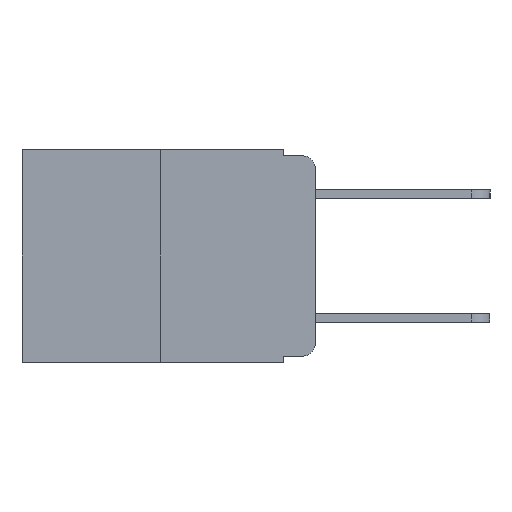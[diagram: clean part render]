
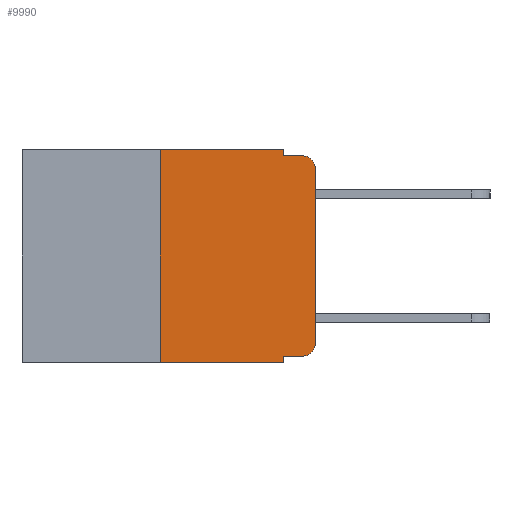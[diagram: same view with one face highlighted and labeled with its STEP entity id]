
A CAD part, left-side view. The second image highlights one B-rep face of the part: STEP entity #9990.
In plain terms, the highlighted planar face has unit normal (-1, 0, 0).
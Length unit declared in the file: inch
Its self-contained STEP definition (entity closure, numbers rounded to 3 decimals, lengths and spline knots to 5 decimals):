
#39 = VECTOR ( 'NONE', #6651, 39.37008 ) ;
#252 = EDGE_CURVE ( 'NONE', #6690, #4127, #8636, .T. ) ;
#424 = ORIENTED_EDGE ( 'NONE', *, *, #975, .F. ) ;
#566 = CARTESIAN_POINT ( 'NONE',  ( 0., 0.051, -0.333 ) ) ;
#813 = VERTEX_POINT ( 'NONE', #3341 ) ;
#815 = CARTESIAN_POINT ( 'NONE',  ( 0., 0.051, -0.343 ) ) ;
#975 = EDGE_CURVE ( 'NONE', #4862, #4857, #8998, .T. ) ;
#1001 = DIRECTION ( 'NONE',  ( 0., 0., -1. ) ) ;
#1686 = CARTESIAN_POINT ( 'NONE',  ( 0., 0.02, -0.01 ) ) ;
#1815 = EDGE_CURVE ( 'NONE', #7677, #4127, #7335, .T. ) ;
#1852 = DIRECTION ( 'NONE',  ( 0., -1., 0. ) ) ;
#1937 = CARTESIAN_POINT ( 'NONE',  ( 0., 0.051, 0. ) ) ;
#2047 = DIRECTION ( 'NONE',  ( 0., -1., 0. ) ) ;
#2063 = VECTOR ( 'NONE', #2047, 39.37008 ) ;
#2156 = CARTESIAN_POINT ( 'NONE',  ( 0., 0.051, -0.01 ) ) ;
#2443 = EDGE_CURVE ( 'NONE', #5878, #5564, #2507, .T. ) ;
#2507 = LINE ( 'NONE', #6646, #39 ) ;
#2585 = ORIENTED_EDGE ( 'NONE', *, *, #8378, .F. ) ;
#2868 = CARTESIAN_POINT ( 'NONE',  ( 0., 0., -0.03 ) ) ;
#2990 = VERTEX_POINT ( 'NONE', #2156 ) ;
#3038 = VERTEX_POINT ( 'NONE', #1686 ) ;
#3105 = AXIS2_PLACEMENT_3D ( 'NONE', #7764, #5228, #10895 ) ;
#3159 = DIRECTION ( 'NONE',  ( 0., 0., 1. ) ) ;
#3266 = CARTESIAN_POINT ( 'NONE',  ( 0., 0.25, 0. ) ) ;
#3341 = CARTESIAN_POINT ( 'NONE',  ( 0., 0.02, -0.333 ) ) ;
#3349 = VECTOR ( 'NONE', #1852, 39.37008 ) ;
#3759 = ORIENTED_EDGE ( 'NONE', *, *, #6313, .T. ) ;
#3770 = CARTESIAN_POINT ( 'NONE',  ( 0., 0.051, -0.01 ) ) ;
#3974 = CARTESIAN_POINT ( 'NONE',  ( 0., 0.051, -0.333 ) ) ;
#4127 = VERTEX_POINT ( 'NONE', #815 ) ;
#4305 = LINE ( 'NONE', #10656, #8768 ) ;
#4346 = EDGE_CURVE ( 'NONE', #6690, #813, #10275, .T. ) ;
#4380 = EDGE_LOOP ( 'NONE', ( #8405, #6462, #4447, #2585, #424, #5248, #9637, #9890, #5779, #3759 ) ) ;
#4447 = ORIENTED_EDGE ( 'NONE', *, *, #6150, .F. ) ;
#4481 = LINE ( 'NONE', #3770, #2063 ) ;
#4497 = CARTESIAN_POINT ( 'NONE',  ( 0., 0.02, -0.03 ) ) ;
#4857 = VERTEX_POINT ( 'NONE', #5536 ) ;
#4862 = VERTEX_POINT ( 'NONE', #9070 ) ;
#5085 = EDGE_CURVE ( 'NONE', #5564, #3038, #6872, .T. ) ;
#5193 = EDGE_CURVE ( 'NONE', #7677, #4862, #8290, .T. ) ;
#5228 = DIRECTION ( 'NONE',  ( 1., 0., 0. ) ) ;
#5248 = ORIENTED_EDGE ( 'NONE', *, *, #5193, .F. ) ;
#5331 = CARTESIAN_POINT ( 'NONE',  ( 0., 0.473, -0.343 ) ) ;
#5333 = VECTOR ( 'NONE', #5379, 39.37008 ) ;
#5379 = DIRECTION ( 'NONE',  ( 0., -1., 0. ) ) ;
#5536 = CARTESIAN_POINT ( 'NONE',  ( 0., 0.051, 0. ) ) ;
#5564 = VERTEX_POINT ( 'NONE', #2868 ) ;
#5629 = DIRECTION ( 'NONE',  ( -1., 0., 0. ) ) ;
#5668 = DIRECTION ( 'NONE',  ( 0., 0., -1. ) ) ;
#5779 = ORIENTED_EDGE ( 'NONE', *, *, #4346, .T. ) ;
#5878 = VERTEX_POINT ( 'NONE', #6399 ) ;
#6150 = EDGE_CURVE ( 'NONE', #2990, #3038, #4481, .T. ) ;
#6313 = EDGE_CURVE ( 'NONE', #813, #5878, #10624, .T. ) ;
#6352 = DIRECTION ( 'NONE',  ( 0., 0., -1. ) ) ;
#6399 = CARTESIAN_POINT ( 'NONE',  ( 0., 0., -0.313 ) ) ;
#6462 = ORIENTED_EDGE ( 'NONE', *, *, #5085, .T. ) ;
#6646 = CARTESIAN_POINT ( 'NONE',  ( 0., 0., 0. ) ) ;
#6651 = DIRECTION ( 'NONE',  ( 0., 0., 1. ) ) ;
#6690 = VERTEX_POINT ( 'NONE', #566 ) ;
#6842 = DIRECTION ( 'NONE',  ( 0., -1., 0. ) ) ;
#6872 = CIRCLE ( 'NONE', #7425, 0.02 ) ;
#7335 = LINE ( 'NONE', #5331, #5333 ) ;
#7425 = AXIS2_PLACEMENT_3D ( 'NONE', #4497, #5629, #5668 ) ;
#7474 = DIRECTION ( 'NONE',  ( 0., 0., -1. ) ) ;
#7558 = DIRECTION ( 'NONE',  ( -1., 0., 0. ) ) ;
#7677 = VERTEX_POINT ( 'NONE', #7778 ) ;
#7745 = FACE_OUTER_BOUND ( 'NONE', #4380, .T. ) ;
#7764 = CARTESIAN_POINT ( 'NONE',  ( 0., 0.473, 0. ) ) ;
#7778 = CARTESIAN_POINT ( 'NONE',  ( 0., 0.25, -0.343 ) ) ;
#7983 = CARTESIAN_POINT ( 'NONE',  ( 0., 0.02, -0.313 ) ) ;
#8051 = VECTOR ( 'NONE', #3159, 39.37008 ) ;
#8290 = LINE ( 'NONE', #3266, #8051 ) ;
#8378 = EDGE_CURVE ( 'NONE', #4857, #2990, #4305, .T. ) ;
#8387 = VECTOR ( 'NONE', #1001, 39.37008 ) ;
#8405 = ORIENTED_EDGE ( 'NONE', *, *, #2443, .T. ) ;
#8636 = LINE ( 'NONE', #1937, #8387 ) ;
#8743 = VECTOR ( 'NONE', #6842, 39.37008 ) ;
#8768 = VECTOR ( 'NONE', #6352, 39.37008 ) ;
#8988 = AXIS2_PLACEMENT_3D ( 'NONE', #7983, #7558, #7474 ) ;
#8998 = LINE ( 'NONE', #9860, #8743 ) ;
#9070 = CARTESIAN_POINT ( 'NONE',  ( 0., 0.25, 0. ) ) ;
#9637 = ORIENTED_EDGE ( 'NONE', *, *, #1815, .T. ) ;
#9860 = CARTESIAN_POINT ( 'NONE',  ( 0., 0.473, 0. ) ) ;
#9890 = ORIENTED_EDGE ( 'NONE', *, *, #252, .F. ) ;
#9990 = ADVANCED_FACE ( 'NONE', ( #7745 ), #10145, .F. ) ;
#10145 = PLANE ( 'NONE',  #3105 ) ;
#10275 = LINE ( 'NONE', #3974, #3349 ) ;
#10624 = CIRCLE ( 'NONE', #8988, 0.02 ) ;
#10656 = CARTESIAN_POINT ( 'NONE',  ( 0., 0.051, 0. ) ) ;
#10895 = DIRECTION ( 'NONE',  ( 0., 0., -1. ) ) ;
